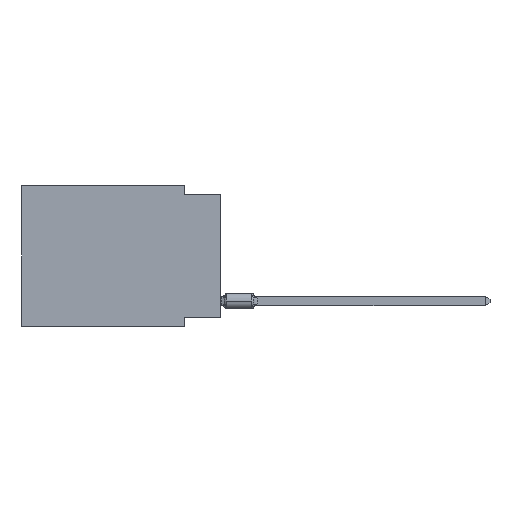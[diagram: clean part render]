
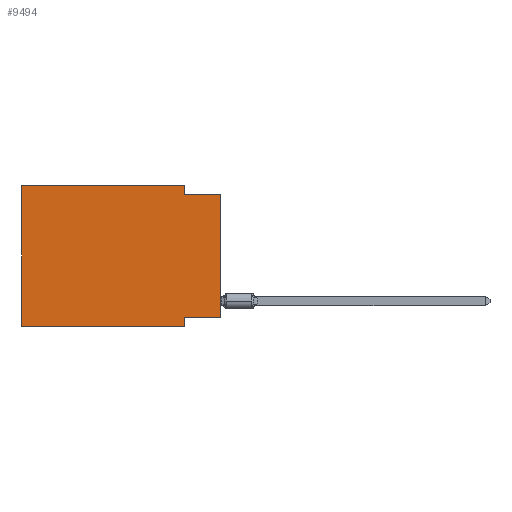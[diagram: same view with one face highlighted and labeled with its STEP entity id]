
A CAD part, left-side view. The second image highlights one B-rep face of the part: STEP entity #9494.
In plain terms, the highlighted planar face has unit normal (-1, 0, 0).
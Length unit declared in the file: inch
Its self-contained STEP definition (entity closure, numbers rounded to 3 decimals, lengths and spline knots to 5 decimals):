
#116 = DIRECTION ( 'NONE',  ( 0., 0., -1. ) ) ;
#483 = LINE ( 'NONE', #45940, #69674 ) ;
#3000 = ORIENTED_EDGE ( 'NONE', *, *, #70343, .F. ) ;
#6335 = EDGE_CURVE ( 'NONE', #43873, #70481, #53568, .T. ) ;
#6603 = LINE ( 'NONE', #69008, #20573 ) ;
#6842 = CARTESIAN_POINT ( 'NONE',  ( 0., 0.1, 0. ) ) ;
#7171 = DIRECTION ( 'NONE',  ( 0., -1., 0. ) ) ;
#7303 = PLANE ( 'NONE',  #37923 ) ;
#7341 = CARTESIAN_POINT ( 'NONE',  ( 0., 0.1, -0.39 ) ) ;
#8619 = VERTEX_POINT ( 'NONE', #50060 ) ;
#9292 = DIRECTION ( 'NONE',  ( 0., 0., -1. ) ) ;
#9494 = ADVANCED_FACE ( 'NONE', ( #57883 ), #7303, .F. ) ;
#9835 = ORIENTED_EDGE ( 'NONE', *, *, #69306, .T. ) ;
#10378 = LINE ( 'NONE', #21460, #51526 ) ;
#11423 = DIRECTION ( 'NONE',  ( 0., -1., 0. ) ) ;
#12120 = CARTESIAN_POINT ( 'NONE',  ( 0., 0.1, -0.365 ) ) ;
#12154 = ORIENTED_EDGE ( 'NONE', *, *, #14994, .F. ) ;
#12273 = EDGE_LOOP ( 'NONE', ( #9835, #40872, #19348, #3000, #70228, #40869, #12154, #12362 ) ) ;
#12362 = ORIENTED_EDGE ( 'NONE', *, *, #27302, .F. ) ;
#12723 = CARTESIAN_POINT ( 'NONE',  ( 0., 0., -0.025 ) ) ;
#14745 = VERTEX_POINT ( 'NONE', #39946 ) ;
#14944 = VERTEX_POINT ( 'NONE', #59464 ) ;
#14994 = EDGE_CURVE ( 'NONE', #19672, #70481, #483, .T. ) ;
#17961 = EDGE_CURVE ( 'NONE', #14745, #70867, #39672, .T. ) ;
#19348 = ORIENTED_EDGE ( 'NONE', *, *, #32141, .F. ) ;
#19672 = VERTEX_POINT ( 'NONE', #12120 ) ;
#20573 = VECTOR ( 'NONE', #29162, 39.37008 ) ;
#21460 = CARTESIAN_POINT ( 'NONE',  ( 0., 0., -0.365 ) ) ;
#21624 = VERTEX_POINT ( 'NONE', #72147 ) ;
#27302 = EDGE_CURVE ( 'NONE', #8619, #19672, #10378, .T. ) ;
#28082 = CARTESIAN_POINT ( 'NONE',  ( 0., 0.55, -0.39 ) ) ;
#29162 = DIRECTION ( 'NONE',  ( 0., 0., 1. ) ) ;
#30572 = DIRECTION ( 'NONE',  ( 0., 0., -1. ) ) ;
#31787 = DIRECTION ( 'NONE',  ( 0., -1., 0. ) ) ;
#32141 = EDGE_CURVE ( 'NONE', #21624, #14745, #70969, .T. ) ;
#33261 = CARTESIAN_POINT ( 'NONE',  ( 0., 0.55, 0. ) ) ;
#37147 = EDGE_CURVE ( 'NONE', #43873, #14944, #61317, .T. ) ;
#37186 = VECTOR ( 'NONE', #9292, 39.37008 ) ;
#37923 = AXIS2_PLACEMENT_3D ( 'NONE', #64512, #46463, #30572 ) ;
#39672 = LINE ( 'NONE', #12723, #46338 ) ;
#39946 = CARTESIAN_POINT ( 'NONE',  ( 0., 0.1, -0.025 ) ) ;
#40289 = DIRECTION ( 'NONE',  ( 0., 1., 0. ) ) ;
#40869 = ORIENTED_EDGE ( 'NONE', *, *, #6335, .T. ) ;
#40872 = ORIENTED_EDGE ( 'NONE', *, *, #17961, .F. ) ;
#43873 = VERTEX_POINT ( 'NONE', #28082 ) ;
#45940 = CARTESIAN_POINT ( 'NONE',  ( 0., 0.1, -0.39 ) ) ;
#46338 = VECTOR ( 'NONE', #7171, 39.37008 ) ;
#46463 = DIRECTION ( 'NONE',  ( 1., 0., 0. ) ) ;
#50060 = CARTESIAN_POINT ( 'NONE',  ( 0., 0., -0.365 ) ) ;
#51361 = VECTOR ( 'NONE', #11423, 39.37008 ) ;
#51526 = VECTOR ( 'NONE', #40289, 39.37008 ) ;
#51739 = VECTOR ( 'NONE', #68348, 39.37008 ) ;
#53568 = LINE ( 'NONE', #70204, #65644 ) ;
#55990 = CARTESIAN_POINT ( 'NONE',  ( 0., 0., -0.025 ) ) ;
#57883 = FACE_OUTER_BOUND ( 'NONE', #12273, .T. ) ;
#59464 = CARTESIAN_POINT ( 'NONE',  ( 0., 0.55, 0. ) ) ;
#61262 = LINE ( 'NONE', #67552, #51361 ) ;
#61317 = LINE ( 'NONE', #33261, #51739 ) ;
#64512 = CARTESIAN_POINT ( 'NONE',  ( 0., 0.55, 0. ) ) ;
#65644 = VECTOR ( 'NONE', #31787, 39.37008 ) ;
#67552 = CARTESIAN_POINT ( 'NONE',  ( 0., 0.55, 0. ) ) ;
#68348 = DIRECTION ( 'NONE',  ( 0., 0., 1. ) ) ;
#69008 = CARTESIAN_POINT ( 'NONE',  ( 0., 0., 0. ) ) ;
#69306 = EDGE_CURVE ( 'NONE', #8619, #70867, #6603, .T. ) ;
#69674 = VECTOR ( 'NONE', #116, 39.37008 ) ;
#70204 = CARTESIAN_POINT ( 'NONE',  ( 0., 0.55, -0.39 ) ) ;
#70228 = ORIENTED_EDGE ( 'NONE', *, *, #37147, .F. ) ;
#70343 = EDGE_CURVE ( 'NONE', #14944, #21624, #61262, .T. ) ;
#70481 = VERTEX_POINT ( 'NONE', #7341 ) ;
#70867 = VERTEX_POINT ( 'NONE', #55990 ) ;
#70969 = LINE ( 'NONE', #6842, #37186 ) ;
#72147 = CARTESIAN_POINT ( 'NONE',  ( 0., 0.1, 0. ) ) ;
